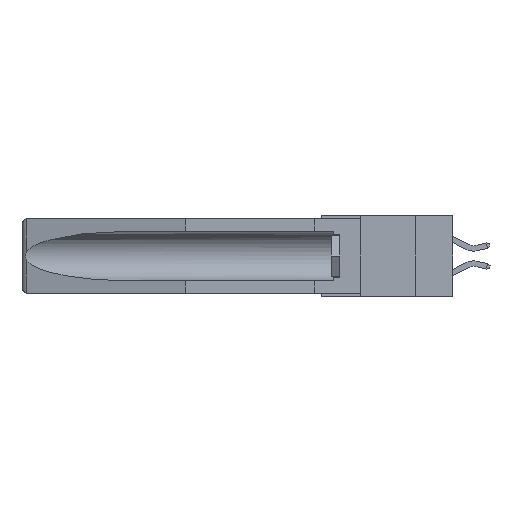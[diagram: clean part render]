
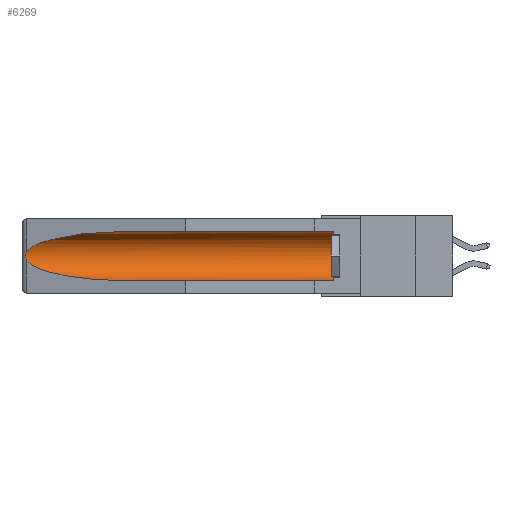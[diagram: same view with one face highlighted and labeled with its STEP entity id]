
A CAD part, left-side view. The second image highlights one B-rep face of the part: STEP entity #6269.
In plain terms, the highlighted cylindrical face has radius 2.857 mm (diameter 5.715 mm), a partial arc.
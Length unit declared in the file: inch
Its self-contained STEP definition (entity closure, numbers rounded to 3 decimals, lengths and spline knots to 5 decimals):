
#319 = DIRECTION ( 'NONE',  ( 0., 1., 0. ) ) ;
#480 = CARTESIAN_POINT ( 'NONE',  ( 0.155, -0.30754, -0.1715 ) ) ;
#923 = CARTESIAN_POINT ( 'NONE',  ( 0.155, 0.126, -0.1715 ) ) ;
#1395 = CYLINDRICAL_SURFACE ( 'NONE', #8174, 0.1125 ) ;
#1688 = CARTESIAN_POINT ( 'NONE',  ( 0.26537, 1.52718, -0.19328 ) ) ;
#1934 = LINE ( 'NONE', #19757, #26126 ) ;
#2198 = CARTESIAN_POINT ( 'NONE',  ( 0.21114, 1.30732, -0.059 ) ) ;
#2614 = DIRECTION ( 'NONE',  ( 0., 0., 1. ) ) ;
#2618 = B_SPLINE_CURVE_WITH_KNOTS ( 'NONE', 3,
 ( #9679, #7435, #14224, #22276, #16259, #3755, #24747, #16691, #16355, #16607 ),
 .UNSPECIFIED., .F., .F.,
 ( 4, 2, 2, 2, 4 ),
 ( 0., 0.00029, 0.00058, 0.00087, 0.00117 ),
 .UNSPECIFIED. ) ;
#3063 = VERTEX_POINT ( 'NONE', #23472 ) ;
#3755 = CARTESIAN_POINT ( 'NONE',  ( 0.2675, 1.53308, -0.17534 ) ) ;
#3949 = FACE_OUTER_BOUND ( 'NONE', #25538, .T. ) ;
#4410 = AXIS2_PLACEMENT_3D ( 'NONE', #923, #23179, #6824 ) ;
#4723 = VERTEX_POINT ( 'NONE', #20800 ) ;
#4884 = CIRCLE ( 'NONE', #4410, 0.1125 ) ;
#6168 =( BOUNDED_CURVE ( )  B_SPLINE_CURVE ( 3, ( #16559, #2198, #20509, #10448 ),
 .UNSPECIFIED., .F., .F. ) 
 B_SPLINE_CURVE_WITH_KNOTS ( ( 4, 4 ),
 ( 4.71239, 6.08839 ),
 .UNSPECIFIED. ) 
 CURVE ( )  GEOMETRIC_REPRESENTATION_ITEM ( )  RATIONAL_B_SPLINE_CURVE ( ( 1., 0.848, 0.848, 1. ) ) 
 REPRESENTATION_ITEM ( '' )  );
#6269 = ADVANCED_FACE ( 'NONE', ( #3949 ), #1395, .F. ) ;
#6824 = DIRECTION ( 'NONE',  ( 0., 0., 1. ) ) ;
#7435 = CARTESIAN_POINT ( 'NONE',  ( 0.26597, 1.52961, -0.15275 ) ) ;
#7912 = EDGE_CURVE ( 'NONE', #3063, #14350, #1934, .T. ) ;
#8174 = AXIS2_PLACEMENT_3D ( 'NONE', #480, #319, #2614 ) ;
#8890 = ORIENTED_EDGE ( 'NONE', *, *, #22221, .T. ) ;
#9679 = CARTESIAN_POINT ( 'NONE',  ( 0.26537, 1.52718, -0.14972 ) ) ;
#10448 = CARTESIAN_POINT ( 'NONE',  ( 0.26537, 1.52718, -0.14972 ) ) ;
#11359 = ORIENTED_EDGE ( 'NONE', *, *, #13947, .T. ) ;
#11786 = CARTESIAN_POINT ( 'NONE',  ( 0.155, 0.126, -0.284 ) ) ;
#12240 = DIRECTION ( 'NONE',  ( 0., 1., 0. ) ) ;
#13728 = ORIENTED_EDGE ( 'NONE', *, *, #7912, .T. ) ;
#13947 = EDGE_CURVE ( 'NONE', #15858, #3063, #4884, .T. ) ;
#14224 = CARTESIAN_POINT ( 'NONE',  ( 0.26654, 1.53092, -0.15636 ) ) ;
#14350 = VERTEX_POINT ( 'NONE', #15810 ) ;
#14432 = EDGE_CURVE ( 'NONE', #4723, #24422, #17600, .T. ) ;
#15723 = CARTESIAN_POINT ( 'NONE',  ( 0.25451, 1.48313, -0.24835 ) ) ;
#15810 = CARTESIAN_POINT ( 'NONE',  ( 0.155, 1.07973, -0.059 ) ) ;
#15858 = VERTEX_POINT ( 'NONE', #11786 ) ;
#16259 = CARTESIAN_POINT ( 'NONE',  ( 0.2675, 1.53308, -0.16763 ) ) ;
#16355 = CARTESIAN_POINT ( 'NONE',  ( 0.26597, 1.5296, -0.19026 ) ) ;
#16559 = CARTESIAN_POINT ( 'NONE',  ( 0.155, 1.07973, -0.059 ) ) ;
#16607 = CARTESIAN_POINT ( 'NONE',  ( 0.26537, 1.52718, -0.19328 ) ) ;
#16691 = CARTESIAN_POINT ( 'NONE',  ( 0.26655, 1.53094, -0.18657 ) ) ;
#16901 = ORIENTED_EDGE ( 'NONE', *, *, #18888, .F. ) ;
#17213 = EDGE_CURVE ( 'NONE', #14350, #25151, #6168, .T. ) ;
#17479 = LINE ( 'NONE', #24528, #22302 ) ;
#17600 =( BOUNDED_CURVE ( )  B_SPLINE_CURVE ( 3, ( #1688, #15723, #19976, #26143 ),
 .UNSPECIFIED., .F., .F. ) 
 B_SPLINE_CURVE_WITH_KNOTS ( ( 4, 4 ),
 ( 0.1948, 1.5708 ),
 .UNSPECIFIED. ) 
 CURVE ( )  GEOMETRIC_REPRESENTATION_ITEM ( )  RATIONAL_B_SPLINE_CURVE ( ( 1., 0.848, 0.848, 1. ) ) 
 REPRESENTATION_ITEM ( '' )  );
#17938 = CARTESIAN_POINT ( 'NONE',  ( 0.155, 1.07973, -0.284 ) ) ;
#18888 = EDGE_CURVE ( 'NONE', #15858, #24422, #17479, .T. ) ;
#19320 = ORIENTED_EDGE ( 'NONE', *, *, #14432, .T. ) ;
#19757 = CARTESIAN_POINT ( 'NONE',  ( 0.155, -0.30754, -0.059 ) ) ;
#19976 = CARTESIAN_POINT ( 'NONE',  ( 0.21114, 1.30732, -0.284 ) ) ;
#20509 = CARTESIAN_POINT ( 'NONE',  ( 0.25451, 1.48313, -0.09465 ) ) ;
#20800 = CARTESIAN_POINT ( 'NONE',  ( 0.26537, 1.52718, -0.19328 ) ) ;
#21440 = CARTESIAN_POINT ( 'NONE',  ( 0.26537, 1.52718, -0.14972 ) ) ;
#22221 = EDGE_CURVE ( 'NONE', #25151, #4723, #2618, .T. ) ;
#22276 = CARTESIAN_POINT ( 'NONE',  ( 0.2673, 1.5327, -0.16383 ) ) ;
#22302 = VECTOR ( 'NONE', #12240, 39.37008 ) ;
#22941 = ORIENTED_EDGE ( 'NONE', *, *, #17213, .T. ) ;
#23179 = DIRECTION ( 'NONE',  ( 0., -1., 0. ) ) ;
#23472 = CARTESIAN_POINT ( 'NONE',  ( 0.155, 0.126, -0.059 ) ) ;
#24146 = DIRECTION ( 'NONE',  ( 0., 1., 0. ) ) ;
#24422 = VERTEX_POINT ( 'NONE', #17938 ) ;
#24528 = CARTESIAN_POINT ( 'NONE',  ( 0.155, -0.30754, -0.284 ) ) ;
#24747 = CARTESIAN_POINT ( 'NONE',  ( 0.2673, 1.53269, -0.17917 ) ) ;
#25151 = VERTEX_POINT ( 'NONE', #21440 ) ;
#25538 = EDGE_LOOP ( 'NONE', ( #22941, #8890, #19320, #16901, #11359, #13728 ) ) ;
#26126 = VECTOR ( 'NONE', #24146, 39.37008 ) ;
#26143 = CARTESIAN_POINT ( 'NONE',  ( 0.155, 1.07973, -0.284 ) ) ;
